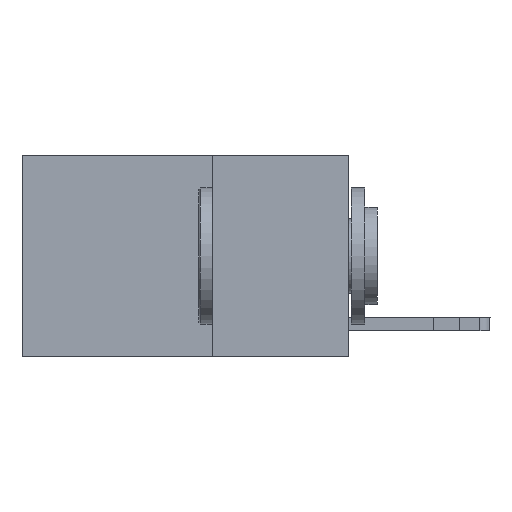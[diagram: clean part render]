
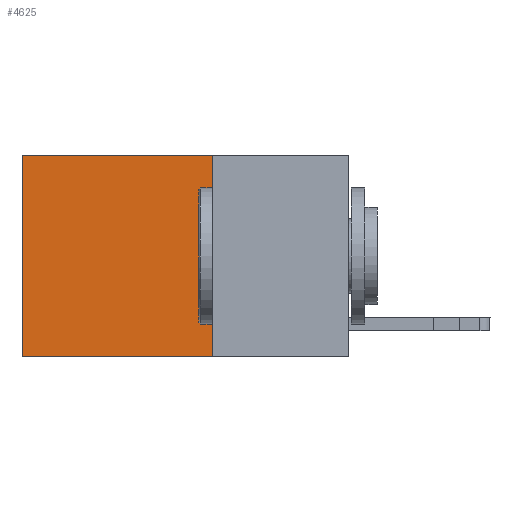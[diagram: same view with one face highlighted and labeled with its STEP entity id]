
A CAD part, left-side view. The second image highlights one B-rep face of the part: STEP entity #4625.
In plain terms, the highlighted planar face has unit normal (-1, 0, 0).
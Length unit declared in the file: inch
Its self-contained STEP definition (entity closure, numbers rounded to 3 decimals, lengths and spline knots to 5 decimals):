
#142 = LINE ( 'NONE', #9877, #11304 ) ;
#205 = ORIENTED_EDGE ( 'NONE', *, *, #5668, .F. ) ;
#1068 = DIRECTION ( 'NONE',  ( 0., 1., 0. ) ) ;
#1838 = DIRECTION ( 'NONE',  ( 0., 0., -1. ) ) ;
#1942 = ORIENTED_EDGE ( 'NONE', *, *, #7317, .T. ) ;
#2323 = EDGE_CURVE ( 'NONE', #10836, #4055, #13287, .T. ) ;
#2702 = LINE ( 'NONE', #5648, #5602 ) ;
#2932 = FACE_OUTER_BOUND ( 'NONE', #10386, .T. ) ;
#3225 = AXIS2_PLACEMENT_3D ( 'NONE', #7042, #11216, #7173 ) ;
#4055 = VERTEX_POINT ( 'NONE', #7518 ) ;
#4291 = DIRECTION ( 'NONE',  ( 0., 1., 0. ) ) ;
#4625 = ADVANCED_FACE ( 'NONE', ( #2932 ), #11442, .F. ) ;
#4741 = VERTEX_POINT ( 'NONE', #11726 ) ;
#5055 = LINE ( 'NONE', #9191, #6871 ) ;
#5602 = VECTOR ( 'NONE', #7778, 39.37008 ) ;
#5648 = CARTESIAN_POINT ( 'NONE',  ( 0.2625, 0.25, 0. ) ) ;
#5668 = EDGE_CURVE ( 'NONE', #4741, #10501, #2702, .T. ) ;
#6494 = EDGE_CURVE ( 'NONE', #10501, #4055, #5055, .T. ) ;
#6766 = CARTESIAN_POINT ( 'NONE',  ( 0.2625, 0.6, 0. ) ) ;
#6871 = VECTOR ( 'NONE', #1068, 39.37008 ) ;
#7042 = CARTESIAN_POINT ( 'NONE',  ( 0.2625, 0.25, 0. ) ) ;
#7058 = CARTESIAN_POINT ( 'NONE',  ( 0.2625, 0.25, -0.37 ) ) ;
#7173 = DIRECTION ( 'NONE',  ( 0., 0., -1. ) ) ;
#7317 = EDGE_CURVE ( 'NONE', #4741, #10836, #142, .T. ) ;
#7518 = CARTESIAN_POINT ( 'NONE',  ( 0.2625, 0.6, -0.37 ) ) ;
#7778 = DIRECTION ( 'NONE',  ( 0., 0., -1. ) ) ;
#8037 = CARTESIAN_POINT ( 'NONE',  ( 0.2625, 0.6, 0. ) ) ;
#9191 = CARTESIAN_POINT ( 'NONE',  ( 0.2625, 0.25, -0.37 ) ) ;
#9369 = ORIENTED_EDGE ( 'NONE', *, *, #6494, .F. ) ;
#9566 = ORIENTED_EDGE ( 'NONE', *, *, #2323, .T. ) ;
#9877 = CARTESIAN_POINT ( 'NONE',  ( 0.2625, 0.25, 0. ) ) ;
#10386 = EDGE_LOOP ( 'NONE', ( #9566, #9369, #205, #1942 ) ) ;
#10501 = VERTEX_POINT ( 'NONE', #7058 ) ;
#10836 = VERTEX_POINT ( 'NONE', #6766 ) ;
#11216 = DIRECTION ( 'NONE',  ( 1., 0., 0. ) ) ;
#11304 = VECTOR ( 'NONE', #4291, 39.37008 ) ;
#11442 = PLANE ( 'NONE',  #3225 ) ;
#11726 = CARTESIAN_POINT ( 'NONE',  ( 0.2625, 0.25, 0. ) ) ;
#12261 = VECTOR ( 'NONE', #1838, 39.37008 ) ;
#13287 = LINE ( 'NONE', #8037, #12261 ) ;
